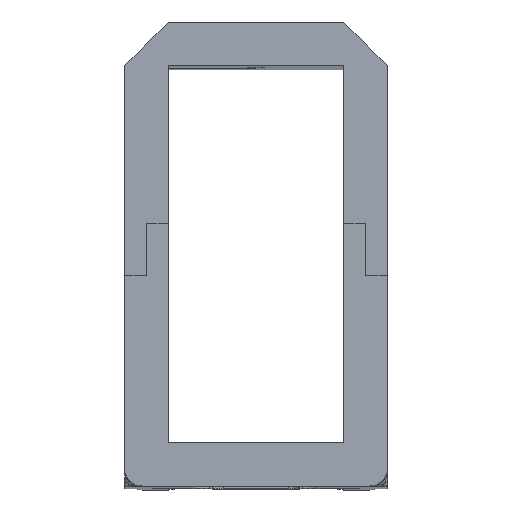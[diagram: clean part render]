
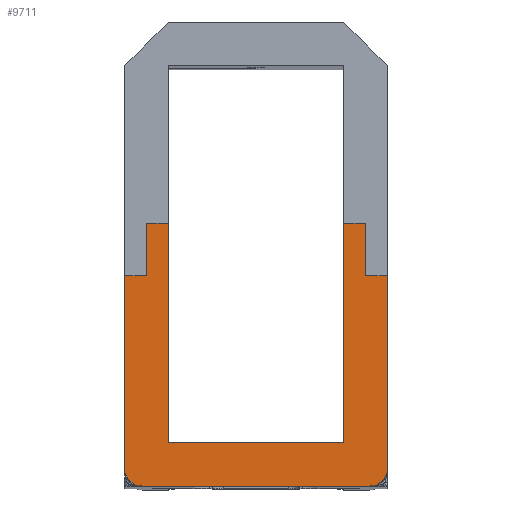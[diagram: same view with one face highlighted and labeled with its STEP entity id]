
A CAD part, top view. The second image highlights one B-rep face of the part: STEP entity #9711.
In plain terms, the highlighted planar face has unit normal (0, 0, 1).
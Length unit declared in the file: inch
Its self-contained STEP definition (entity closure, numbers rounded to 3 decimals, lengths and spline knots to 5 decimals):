
#15 = VERTEX_POINT ( 'NONE', #12178 ) ;
#50 = ORIENTED_EDGE ( 'NONE', *, *, #7093, .T. ) ;
#63 = EDGE_CURVE ( 'NONE', #11046, #9485, #1314, .T. ) ;
#159 = CARTESIAN_POINT ( 'NONE',  ( 1.4, 0., 16.5 ) ) ;
#209 = VERTEX_POINT ( 'NONE', #700 ) ;
#418 = ORIENTED_EDGE ( 'NONE', *, *, #5517, .F. ) ;
#481 = DIRECTION ( 'NONE',  ( 1., 0., 0. ) ) ;
#672 = LINE ( 'NONE', #8513, #1417 ) ;
#700 = CARTESIAN_POINT ( 'NONE',  ( 1.25, 0.25, 16.5 ) ) ;
#728 = CARTESIAN_POINT ( 'NONE',  ( 0., 0.1, 16.5 ) ) ;
#1005 = DIRECTION ( 'NONE',  ( -1., 0., 0. ) ) ;
#1025 = CARTESIAN_POINT ( 'NONE',  ( 0., 0., 16.5 ) ) ;
#1044 = ORIENTED_EDGE ( 'NONE', *, *, #4850, .T. ) ;
#1154 = DIRECTION ( 'NONE',  ( 1., 0., 0. ) ) ;
#1314 = LINE ( 'NONE', #3318, #2806 ) ;
#1417 = VECTOR ( 'NONE', #12411, 39.37008 ) ;
#1477 = CARTESIAN_POINT ( 'NONE',  ( 1.5, 1.2, 16.5 ) ) ;
#1623 = VERTEX_POINT ( 'NONE', #8733 ) ;
#1731 = LINE ( 'NONE', #10640, #12181 ) ;
#1809 = AXIS2_PLACEMENT_3D ( 'NONE', #9949, #10910, #1005 ) ;
#1940 = LINE ( 'NONE', #4924, #4619 ) ;
#2644 = ORIENTED_EDGE ( 'NONE', *, *, #5270, .T. ) ;
#2664 = CARTESIAN_POINT ( 'NONE',  ( 0., 0., 16.5 ) ) ;
#2708 = VERTEX_POINT ( 'NONE', #159 ) ;
#2806 = VECTOR ( 'NONE', #4167, 39.37008 ) ;
#2851 = CIRCLE ( 'NONE', #1809, 0.1 ) ;
#3101 = PLANE ( 'NONE',  #6681 ) ;
#3304 = DIRECTION ( 'NONE',  ( 0., -1., 0. ) ) ;
#3318 = CARTESIAN_POINT ( 'NONE',  ( 1.375, 1.5, 16.5 ) ) ;
#3492 = DIRECTION ( 'NONE',  ( 0., -1., 0. ) ) ;
#3864 = DIRECTION ( 'NONE',  ( 0., 1., 0. ) ) ;
#3868 = ORIENTED_EDGE ( 'NONE', *, *, #11728, .F. ) ;
#4082 = DIRECTION ( 'NONE',  ( 0., 0., 1. ) ) ;
#4092 = VECTOR ( 'NONE', #7408, 39.37008 ) ;
#4167 = DIRECTION ( 'NONE',  ( -1., 0., 0. ) ) ;
#4415 = DIRECTION ( 'NONE',  ( -1., 0., 0. ) ) ;
#4425 = VECTOR ( 'NONE', #3492, 39.37008 ) ;
#4455 = ORIENTED_EDGE ( 'NONE', *, *, #12027, .T. ) ;
#4619 = VECTOR ( 'NONE', #8918, 39.37008 ) ;
#4740 = VERTEX_POINT ( 'NONE', #6262 ) ;
#4850 = EDGE_CURVE ( 'NONE', #9537, #9542, #1731, .T. ) ;
#4924 = CARTESIAN_POINT ( 'NONE',  ( 0., -0.00839, 16.5 ) ) ;
#5059 = ORIENTED_EDGE ( 'NONE', *, *, #9802, .T. ) ;
#5265 = CARTESIAN_POINT ( 'NONE',  ( 1.25, 1.5, 16.5 ) ) ;
#5270 = EDGE_CURVE ( 'NONE', #2708, #1623, #6778, .T. ) ;
#5342 = VECTOR ( 'NONE', #6410, 39.37008 ) ;
#5369 = CARTESIAN_POINT ( 'NONE',  ( 0., 1.2, 16.5 ) ) ;
#5417 = VECTOR ( 'NONE', #3864, 39.37008 ) ;
#5449 = CARTESIAN_POINT ( 'NONE',  ( 0.125, 1.5, 16.5 ) ) ;
#5517 = EDGE_CURVE ( 'NONE', #2708, #15, #11570, .T. ) ;
#5678 = DIRECTION ( 'NONE',  ( 0., 1., 0. ) ) ;
#5733 = EDGE_CURVE ( 'NONE', #11310, #15, #2851, .T. ) ;
#5752 = VERTEX_POINT ( 'NONE', #7187 ) ;
#6262 = CARTESIAN_POINT ( 'NONE',  ( 0.125, 1.2, 16.5 ) ) ;
#6410 = DIRECTION ( 'NONE',  ( -1., 0., 0. ) ) ;
#6416 = CARTESIAN_POINT ( 'NONE',  ( 1.25, 1.5, 16.5 ) ) ;
#6430 = ORIENTED_EDGE ( 'NONE', *, *, #11012, .T. ) ;
#6491 = VECTOR ( 'NONE', #9829, 39.37008 ) ;
#6681 = AXIS2_PLACEMENT_3D ( 'NONE', #1025, #4082, #1154 ) ;
#6778 = CIRCLE ( 'NONE', #10954, 0.1 ) ;
#6784 = LINE ( 'NONE', #11865, #5417 ) ;
#7093 = EDGE_CURVE ( 'NONE', #8255, #11046, #672, .T. ) ;
#7101 = EDGE_CURVE ( 'NONE', #12390, #8255, #8635, .T. ) ;
#7187 = CARTESIAN_POINT ( 'NONE',  ( 0., 1.2, 16.5 ) ) ;
#7408 = DIRECTION ( 'NONE',  ( -1., 0., 0. ) ) ;
#7411 = LINE ( 'NONE', #5449, #9855 ) ;
#7470 = CARTESIAN_POINT ( 'NONE',  ( 1.5, 1.2, 16.5 ) ) ;
#7707 = EDGE_LOOP ( 'NONE', ( #6430, #8504, #50, #11953, #4455, #12504, #1044, #5059, #8557, #12139, #3868, #11533, #418, #2644 ) ) ;
#8255 = VERTEX_POINT ( 'NONE', #9844 ) ;
#8454 = LINE ( 'NONE', #6416, #4425 ) ;
#8504 = ORIENTED_EDGE ( 'NONE', *, *, #7101, .T. ) ;
#8513 = CARTESIAN_POINT ( 'NONE',  ( 1.375, 1.2, 16.5 ) ) ;
#8557 = ORIENTED_EDGE ( 'NONE', *, *, #10679, .T. ) ;
#8576 = VECTOR ( 'NONE', #481, 39.37008 ) ;
#8635 = LINE ( 'NONE', #7470, #5342 ) ;
#8665 = CARTESIAN_POINT ( 'NONE',  ( 0.25, 0.25, 16.5 ) ) ;
#8733 = CARTESIAN_POINT ( 'NONE',  ( 1.5, 0.1, 16.5 ) ) ;
#8918 = DIRECTION ( 'NONE',  ( 0., 1., 0. ) ) ;
#9485 = VERTEX_POINT ( 'NONE', #5265 ) ;
#9537 = VERTEX_POINT ( 'NONE', #8665 ) ;
#9542 = VERTEX_POINT ( 'NONE', #11588 ) ;
#9700 = CARTESIAN_POINT ( 'NONE',  ( 1.4, 0.1, 16.5 ) ) ;
#9711 = ADVANCED_FACE ( 'NONE', ( #10869 ), #3101, .T. ) ;
#9802 = EDGE_CURVE ( 'NONE', #9542, #9870, #12230, .T. ) ;
#9826 = VECTOR ( 'NONE', #4415, 39.37008 ) ;
#9829 = DIRECTION ( 'NONE',  ( -1., 0., 0. ) ) ;
#9844 = CARTESIAN_POINT ( 'NONE',  ( 1.375, 1.2, 16.5 ) ) ;
#9855 = VECTOR ( 'NONE', #3304, 39.37008 ) ;
#9870 = VERTEX_POINT ( 'NONE', #12559 ) ;
#9949 = CARTESIAN_POINT ( 'NONE',  ( 0.1, 0.1, 16.5 ) ) ;
#10119 = EDGE_CURVE ( 'NONE', #5752, #4740, #12214, .T. ) ;
#10640 = CARTESIAN_POINT ( 'NONE',  ( 0.25, 0.25, 16.5 ) ) ;
#10679 = EDGE_CURVE ( 'NONE', #9870, #4740, #7411, .T. ) ;
#10701 = CARTESIAN_POINT ( 'NONE',  ( 1.375, 1.5, 16.5 ) ) ;
#10869 = FACE_OUTER_BOUND ( 'NONE', #7707, .T. ) ;
#10910 = DIRECTION ( 'NONE',  ( 0., 0., 1. ) ) ;
#10927 = DIRECTION ( 'NONE',  ( -1., 0., 0. ) ) ;
#10954 = AXIS2_PLACEMENT_3D ( 'NONE', #9700, #12829, #10927 ) ;
#11012 = EDGE_CURVE ( 'NONE', #1623, #12390, #6784, .T. ) ;
#11046 = VERTEX_POINT ( 'NONE', #10701 ) ;
#11310 = VERTEX_POINT ( 'NONE', #728 ) ;
#11533 = ORIENTED_EDGE ( 'NONE', *, *, #5733, .T. ) ;
#11570 = LINE ( 'NONE', #2664, #4092 ) ;
#11588 = CARTESIAN_POINT ( 'NONE',  ( 0.25, 1.5, 16.5 ) ) ;
#11725 = EDGE_CURVE ( 'NONE', #209, #9537, #11842, .T. ) ;
#11728 = EDGE_CURVE ( 'NONE', #11310, #5752, #1940, .T. ) ;
#11842 = LINE ( 'NONE', #12702, #6491 ) ;
#11865 = CARTESIAN_POINT ( 'NONE',  ( 1.5, 0., 16.5 ) ) ;
#11953 = ORIENTED_EDGE ( 'NONE', *, *, #63, .T. ) ;
#12027 = EDGE_CURVE ( 'NONE', #9485, #209, #8454, .T. ) ;
#12139 = ORIENTED_EDGE ( 'NONE', *, *, #10119, .F. ) ;
#12178 = CARTESIAN_POINT ( 'NONE',  ( 0.1, 0., 16.5 ) ) ;
#12181 = VECTOR ( 'NONE', #5678, 39.37008 ) ;
#12214 = LINE ( 'NONE', #5369, #8576 ) ;
#12230 = LINE ( 'NONE', #12355, #9826 ) ;
#12355 = CARTESIAN_POINT ( 'NONE',  ( 0.25, 1.5, 16.5 ) ) ;
#12390 = VERTEX_POINT ( 'NONE', #1477 ) ;
#12411 = DIRECTION ( 'NONE',  ( 0., 1., 0. ) ) ;
#12504 = ORIENTED_EDGE ( 'NONE', *, *, #11725, .T. ) ;
#12559 = CARTESIAN_POINT ( 'NONE',  ( 0.125, 1.5, 16.5 ) ) ;
#12702 = CARTESIAN_POINT ( 'NONE',  ( 1.25, 0.25, 16.5 ) ) ;
#12829 = DIRECTION ( 'NONE',  ( 0., 0., 1. ) ) ;
